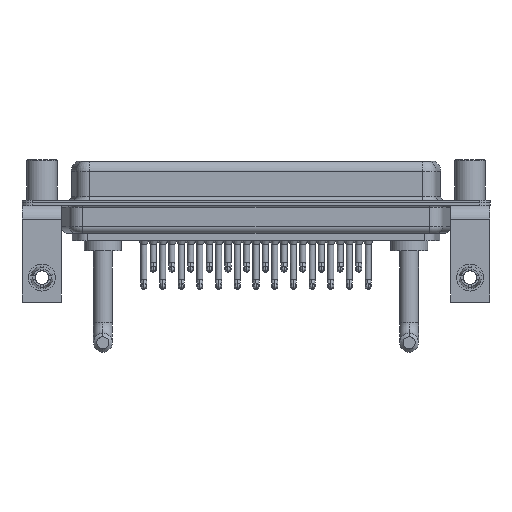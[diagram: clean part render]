
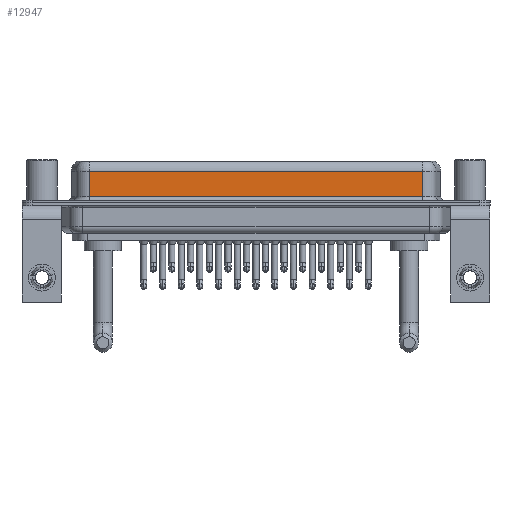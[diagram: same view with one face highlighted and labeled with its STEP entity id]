
A CAD part, front view. The second image highlights one B-rep face of the part: STEP entity #12947.
In plain terms, the highlighted planar face has unit normal (0, -1, 0).
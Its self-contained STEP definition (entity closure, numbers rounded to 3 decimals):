
#25 = EDGE_CURVE ( 'NONE', #19212, #5576, #1736, .T. ) ;
#516 = DIRECTION ( 'NONE',  ( 0., 0., -1. ) ) ;
#1736 = LINE ( 'NONE', #5867, #26256 ) ;
#2494 = EDGE_LOOP ( 'NONE', ( #11139, #25975, #6067, #22071 ) ) ;
#2727 = CARTESIAN_POINT ( 'NONE',  ( 7.038, -3.95, 6.4 ) ) ;
#3166 = EDGE_CURVE ( 'NONE', #18829, #9756, #8457, .T. ) ;
#3981 = VECTOR ( 'NONE', #10134, 1000. ) ;
#4489 = LINE ( 'NONE', #2727, #25046 ) ;
#4978 = AXIS2_PLACEMENT_3D ( 'NONE', #18537, #18973, #5541 ) ;
#5541 = DIRECTION ( 'NONE',  ( 0., 0., 1. ) ) ;
#5576 = VERTEX_POINT ( 'NONE', #21263 ) ;
#5867 = CARTESIAN_POINT ( 'NONE',  ( 56.462, -3.95, 4.65 ) ) ;
#6067 = ORIENTED_EDGE ( 'NONE', *, *, #8958, .T. ) ;
#8084 = CARTESIAN_POINT ( 'NONE',  ( 7.038, -3.95, 0.9 ) ) ;
#8457 = LINE ( 'NONE', #13107, #19770 ) ;
#8958 = EDGE_CURVE ( 'NONE', #5576, #18829, #4489, .T. ) ;
#9756 = VERTEX_POINT ( 'NONE', #13015 ) ;
#10070 = FACE_OUTER_BOUND ( 'NONE', #2494, .T. ) ;
#10134 = DIRECTION ( 'NONE',  ( 0., 0., -1. ) ) ;
#11139 = ORIENTED_EDGE ( 'NONE', *, *, #11906, .F. ) ;
#11906 = EDGE_CURVE ( 'NONE', #19212, #9756, #27839, .T. ) ;
#12947 = ADVANCED_FACE ( 'NONE', ( #10070 ), #25565, .F. ) ;
#13015 = CARTESIAN_POINT ( 'NONE',  ( 56.462, -3.95, 0.9 ) ) ;
#13107 = CARTESIAN_POINT ( 'NONE',  ( 56.462, -3.95, 0.9 ) ) ;
#14873 = DIRECTION ( 'NONE',  ( 1., 0., 0. ) ) ;
#18537 = CARTESIAN_POINT ( 'NONE',  ( 56.462, -3.95, 6.4 ) ) ;
#18829 = VERTEX_POINT ( 'NONE', #8084 ) ;
#18973 = DIRECTION ( 'NONE',  ( 0., 1., 0. ) ) ;
#19212 = VERTEX_POINT ( 'NONE', #21064 ) ;
#19770 = VECTOR ( 'NONE', #14873, 1000. ) ;
#21064 = CARTESIAN_POINT ( 'NONE',  ( 56.462, -3.95, 4.65 ) ) ;
#21263 = CARTESIAN_POINT ( 'NONE',  ( 7.038, -3.95, 4.65 ) ) ;
#21391 = CARTESIAN_POINT ( 'NONE',  ( 56.462, -3.95, 6.4 ) ) ;
#22071 = ORIENTED_EDGE ( 'NONE', *, *, #3166, .T. ) ;
#25046 = VECTOR ( 'NONE', #516, 1000. ) ;
#25565 = PLANE ( 'NONE',  #4978 ) ;
#25975 = ORIENTED_EDGE ( 'NONE', *, *, #25, .T. ) ;
#26256 = VECTOR ( 'NONE', #26472, 1000. ) ;
#26472 = DIRECTION ( 'NONE',  ( -1., 0., 0. ) ) ;
#27839 = LINE ( 'NONE', #21391, #3981 ) ;
